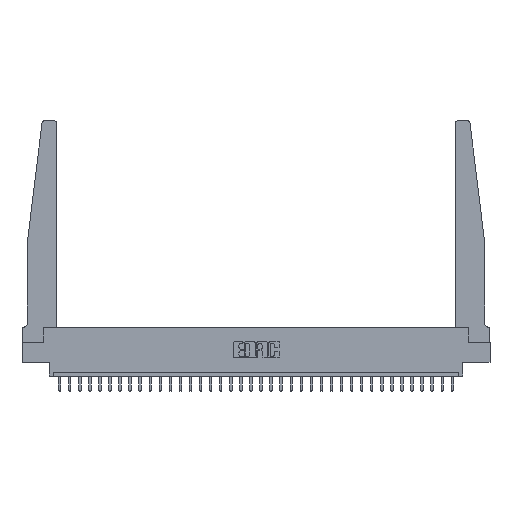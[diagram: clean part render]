
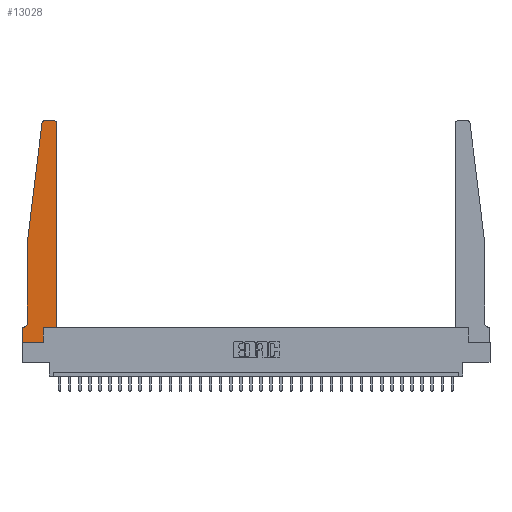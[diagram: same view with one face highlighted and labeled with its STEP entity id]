
A CAD part, top view. The second image highlights one B-rep face of the part: STEP entity #13028.
In plain terms, the highlighted planar face has unit normal (0, 0, 1).
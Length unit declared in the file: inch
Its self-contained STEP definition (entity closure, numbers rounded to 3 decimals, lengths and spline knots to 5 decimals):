
#368 = LINE ( 'NONE', #27655, #14588 ) ;
#370 = EDGE_CURVE ( 'NONE', #28451, #26968, #16936, .T. ) ;
#432 = CARTESIAN_POINT ( 'NONE',  ( 0., 0.1875, 0.37 ) ) ;
#750 = LINE ( 'NONE', #5991, #12434 ) ;
#1588 = VERTEX_POINT ( 'NONE', #21959 ) ;
#1950 = CARTESIAN_POINT ( 'NONE',  ( 0.2605, 0.18, 0.37 ) ) ;
#2241 = CIRCLE ( 'NONE', #2593, 0.05 ) ;
#2593 = AXIS2_PLACEMENT_3D ( 'NONE', #2865, #23802, #10055 ) ;
#2865 = CARTESIAN_POINT ( 'NONE',  ( 0.015, 0.2375, 0.37 ) ) ;
#3127 = DIRECTION ( 'NONE',  ( 0., 0., 1. ) ) ;
#3391 = VERTEX_POINT ( 'NONE', #8726 ) ;
#3741 = ORIENTED_EDGE ( 'NONE', *, *, #7472, .T. ) ;
#3800 = ORIENTED_EDGE ( 'NONE', *, *, #12114, .T. ) ;
#3813 = ORIENTED_EDGE ( 'NONE', *, *, #28796, .T. ) ;
#4769 = EDGE_CURVE ( 'NONE', #15571, #14046, #16860, .T. ) ;
#4907 = EDGE_CURVE ( 'NONE', #14046, #27952, #2241, .T. ) ;
#5012 = PLANE ( 'NONE',  #19890 ) ;
#5566 = ORIENTED_EDGE ( 'NONE', *, *, #11451, .T. ) ;
#5991 = CARTESIAN_POINT ( 'NONE',  ( 0.425, 0.18, 0.37 ) ) ;
#6291 = EDGE_CURVE ( 'NONE', #26023, #3391, #368, .T. ) ;
#6909 = VERTEX_POINT ( 'NONE', #13799 ) ;
#7149 = EDGE_LOOP ( 'NONE', ( #9909, #18173, #13112, #16302, #19668, #12795, #8396, #3800, #3813, #3741, #5566, #7949 ) ) ;
#7269 = CIRCLE ( 'NONE', #21642, 0.03 ) ;
#7472 = EDGE_CURVE ( 'NONE', #14403, #7695, #10860, .T. ) ;
#7590 = DIRECTION ( 'NONE',  ( 0., 0., 1. ) ) ;
#7695 = VERTEX_POINT ( 'NONE', #21512 ) ;
#7949 = ORIENTED_EDGE ( 'NONE', *, *, #27801, .T. ) ;
#8073 = DIRECTION ( 'NONE',  ( 1., 0., 0. ) ) ;
#8320 = CARTESIAN_POINT ( 'NONE',  ( 0.27653, 2.72, 0.37 ) ) ;
#8396 = ORIENTED_EDGE ( 'NONE', *, *, #370, .T. ) ;
#8726 = CARTESIAN_POINT ( 'NONE',  ( 0.27653, 2.75, 0.37 ) ) ;
#9018 = CARTESIAN_POINT ( 'NONE',  ( 0., 0., 0.37 ) ) ;
#9603 = VECTOR ( 'NONE', #20578, 39.37008 ) ;
#9909 = ORIENTED_EDGE ( 'NONE', *, *, #6291, .T. ) ;
#10055 = DIRECTION ( 'NONE',  ( -1., 0., 0. ) ) ;
#10602 = CARTESIAN_POINT ( 'NONE',  ( 0.015, 0.1875, 0.37 ) ) ;
#10860 = LINE ( 'NONE', #22872, #13778 ) ;
#10939 = DIRECTION ( 'NONE',  ( 1., 0., 0. ) ) ;
#11296 = DIRECTION ( 'NONE',  ( 0., -1., 0. ) ) ;
#11377 = DIRECTION ( 'NONE',  ( 0., 1., 0. ) ) ;
#11451 = EDGE_CURVE ( 'NONE', #7695, #1588, #750, .T. ) ;
#11479 = CARTESIAN_POINT ( 'NONE',  ( 0., 0., 0.37 ) ) ;
#11806 = AXIS2_PLACEMENT_3D ( 'NONE', #8320, #7590, #22288 ) ;
#12114 = EDGE_CURVE ( 'NONE', #26968, #28679, #24344, .T. ) ;
#12434 = VECTOR ( 'NONE', #16585, 39.37008 ) ;
#12795 = ORIENTED_EDGE ( 'NONE', *, *, #17007, .T. ) ;
#12866 = VECTOR ( 'NONE', #11377, 39.37008 ) ;
#13028 = ADVANCED_FACE ( 'NONE', ( #19210 ), #5012, .T. ) ;
#13112 = ORIENTED_EDGE ( 'NONE', *, *, #28032, .T. ) ;
#13482 = VECTOR ( 'NONE', #10939, 39.37008 ) ;
#13502 = CARTESIAN_POINT ( 'NONE',  ( 0.065, 1.25, 0.37 ) ) ;
#13778 = VECTOR ( 'NONE', #25197, 39.37008 ) ;
#13799 = CARTESIAN_POINT ( 'NONE',  ( 0.24675, 2.72367, 0.37 ) ) ;
#14046 = VERTEX_POINT ( 'NONE', #17803 ) ;
#14403 = VERTEX_POINT ( 'NONE', #25486 ) ;
#14588 = VECTOR ( 'NONE', #23641, 39.37008 ) ;
#14938 = VECTOR ( 'NONE', #26851, 39.37008 ) ;
#15170 = CARTESIAN_POINT ( 'NONE',  ( 0.065, 1.25, 0.37 ) ) ;
#15571 = VERTEX_POINT ( 'NONE', #13502 ) ;
#15987 = DIRECTION ( 'NONE',  ( -0.122, -0.992, 0. ) ) ;
#16258 = CIRCLE ( 'NONE', #11806, 0.03 ) ;
#16302 = ORIENTED_EDGE ( 'NONE', *, *, #4769, .T. ) ;
#16483 = LINE ( 'NONE', #15170, #21884 ) ;
#16585 = DIRECTION ( 'NONE',  ( 0., 1., 0. ) ) ;
#16860 = LINE ( 'NONE', #18197, #9603 ) ;
#16936 = LINE ( 'NONE', #17875, #27460 ) ;
#17007 = EDGE_CURVE ( 'NONE', #27952, #28451, #23598, .T. ) ;
#17803 = CARTESIAN_POINT ( 'NONE',  ( 0.065, 0.2375, 0.37 ) ) ;
#17865 = CARTESIAN_POINT ( 'NONE',  ( 0.2605, 0., 0.37 ) ) ;
#17875 = CARTESIAN_POINT ( 'NONE',  ( 0., 0., 0.37 ) ) ;
#18173 = ORIENTED_EDGE ( 'NONE', *, *, #19686, .T. ) ;
#18197 = CARTESIAN_POINT ( 'NONE',  ( 0.065, 1.25, 0.37 ) ) ;
#19210 = FACE_OUTER_BOUND ( 'NONE', #7149, .T. ) ;
#19483 = CARTESIAN_POINT ( 'NONE',  ( 0., 0.1875, 0.37 ) ) ;
#19668 = ORIENTED_EDGE ( 'NONE', *, *, #4907, .T. ) ;
#19686 = EDGE_CURVE ( 'NONE', #3391, #6909, #16258, .T. ) ;
#19890 = AXIS2_PLACEMENT_3D ( 'NONE', #432, #21367, #26039 ) ;
#20578 = DIRECTION ( 'NONE',  ( 0., -1., 0. ) ) ;
#21367 = DIRECTION ( 'NONE',  ( 0., 0., 1. ) ) ;
#21403 = CARTESIAN_POINT ( 'NONE',  ( 0.395, 2.75, 0.37 ) ) ;
#21512 = CARTESIAN_POINT ( 'NONE',  ( 0.425, 0.18, 0.37 ) ) ;
#21642 = AXIS2_PLACEMENT_3D ( 'NONE', #28747, #3127, #8073 ) ;
#21884 = VECTOR ( 'NONE', #15987, 39.37008 ) ;
#21959 = CARTESIAN_POINT ( 'NONE',  ( 0.425, 2.72, 0.37 ) ) ;
#22193 = CARTESIAN_POINT ( 'NONE',  ( 0.065, 0.1875, 0.37 ) ) ;
#22288 = DIRECTION ( 'NONE',  ( 1., 0., 0. ) ) ;
#22872 = CARTESIAN_POINT ( 'NONE',  ( 0.425, 0.18, 0.37 ) ) ;
#23598 = LINE ( 'NONE', #22193, #14938 ) ;
#23641 = DIRECTION ( 'NONE',  ( -1., 0., 0. ) ) ;
#23802 = DIRECTION ( 'NONE',  ( 0., 0., -1. ) ) ;
#24344 = LINE ( 'NONE', #11479, #13482 ) ;
#24805 = LINE ( 'NONE', #1950, #12866 ) ;
#25197 = DIRECTION ( 'NONE',  ( 1., 0., 0. ) ) ;
#25486 = CARTESIAN_POINT ( 'NONE',  ( 0.2605, 0.18, 0.37 ) ) ;
#26023 = VERTEX_POINT ( 'NONE', #21403 ) ;
#26039 = DIRECTION ( 'NONE',  ( 1., 0., 0. ) ) ;
#26851 = DIRECTION ( 'NONE',  ( -1., 0., 0. ) ) ;
#26968 = VERTEX_POINT ( 'NONE', #9018 ) ;
#27460 = VECTOR ( 'NONE', #11296, 39.37008 ) ;
#27655 = CARTESIAN_POINT ( 'NONE',  ( 0.25, 2.75, 0.37 ) ) ;
#27801 = EDGE_CURVE ( 'NONE', #1588, #26023, #7269, .T. ) ;
#27952 = VERTEX_POINT ( 'NONE', #10602 ) ;
#28032 = EDGE_CURVE ( 'NONE', #6909, #15571, #16483, .T. ) ;
#28451 = VERTEX_POINT ( 'NONE', #19483 ) ;
#28679 = VERTEX_POINT ( 'NONE', #17865 ) ;
#28747 = CARTESIAN_POINT ( 'NONE',  ( 0.395, 2.72, 0.37 ) ) ;
#28796 = EDGE_CURVE ( 'NONE', #28679, #14403, #24805, .T. ) ;
